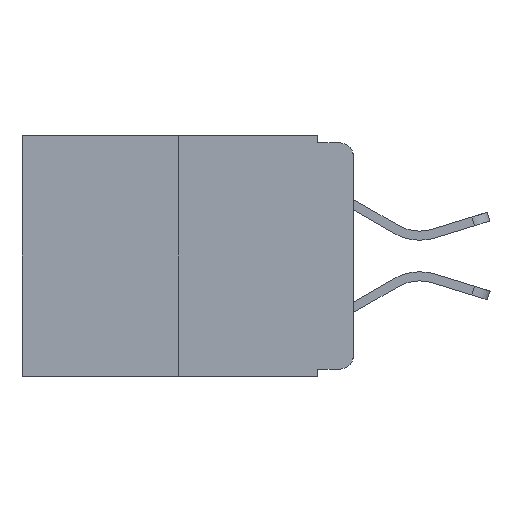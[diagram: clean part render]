
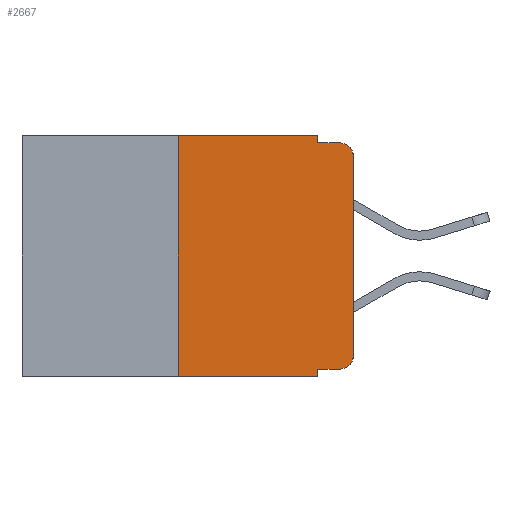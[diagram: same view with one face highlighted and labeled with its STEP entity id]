
A CAD part, left-side view. The second image highlights one B-rep face of the part: STEP entity #2667.
In plain terms, the highlighted planar face has unit normal (-1, 0, 0).
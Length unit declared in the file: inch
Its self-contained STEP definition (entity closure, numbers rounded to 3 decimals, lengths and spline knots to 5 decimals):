
#70 = ORIENTED_EDGE ( 'NONE', *, *, #11704, .T. ) ;
#273 = DIRECTION ( 'NONE',  ( -1., 0., 0. ) ) ;
#379 = CARTESIAN_POINT ( 'NONE',  ( 0., 0.02, -0.03 ) ) ;
#642 = CARTESIAN_POINT ( 'NONE',  ( 0., 0.051, -0.01 ) ) ;
#656 = LINE ( 'NONE', #13604, #9080 ) ;
#787 = CARTESIAN_POINT ( 'NONE',  ( 0., 0.25, -0.343 ) ) ;
#1092 = DIRECTION ( 'NONE',  ( 0., 0., -1. ) ) ;
#2587 = CARTESIAN_POINT ( 'NONE',  ( 0., 0.051, 0. ) ) ;
#2667 = ADVANCED_FACE ( 'NONE', ( #18910 ), #13984, .F. ) ;
#2803 = LINE ( 'NONE', #11101, #20347 ) ;
#3010 = LINE ( 'NONE', #6108, #13708 ) ;
#4211 = DIRECTION ( 'NONE',  ( 0., -1., 0. ) ) ;
#4557 = ORIENTED_EDGE ( 'NONE', *, *, #12743, .T. ) ;
#5712 = EDGE_CURVE ( 'NONE', #15341, #13823, #3010, .T. ) ;
#5773 = AXIS2_PLACEMENT_3D ( 'NONE', #379, #273, #9454 ) ;
#5851 = DIRECTION ( 'NONE',  ( 0., -1., 0. ) ) ;
#5857 = CARTESIAN_POINT ( 'NONE',  ( 0., 0., 0. ) ) ;
#6027 = DIRECTION ( 'NONE',  ( 1., 0., 0. ) ) ;
#6108 = CARTESIAN_POINT ( 'NONE',  ( 0., 0.051, 0. ) ) ;
#6131 = VECTOR ( 'NONE', #11629, 39.37008 ) ;
#6478 = CARTESIAN_POINT ( 'NONE',  ( 0., 0.051, 0. ) ) ;
#7147 = CIRCLE ( 'NONE', #5773, 0.02 ) ;
#7428 = CARTESIAN_POINT ( 'NONE',  ( 0., 0.051, -0.333 ) ) ;
#7812 = VERTEX_POINT ( 'NONE', #8791 ) ;
#8414 = VERTEX_POINT ( 'NONE', #18873 ) ;
#8791 = CARTESIAN_POINT ( 'NONE',  ( 0., 0.25, 0. ) ) ;
#8841 = EDGE_CURVE ( 'NONE', #7812, #15341, #656, .T. ) ;
#9080 = VECTOR ( 'NONE', #5851, 39.37008 ) ;
#9187 = DIRECTION ( 'NONE',  ( 0., 0., -1. ) ) ;
#9247 = LINE ( 'NONE', #5857, #9453 ) ;
#9311 = CARTESIAN_POINT ( 'NONE',  ( 0., 0.051, -0.343 ) ) ;
#9453 = VECTOR ( 'NONE', #15525, 39.37008 ) ;
#9454 = DIRECTION ( 'NONE',  ( 0., 0., -1. ) ) ;
#9625 = VERTEX_POINT ( 'NONE', #787 ) ;
#9995 = LINE ( 'NONE', #642, #15996 ) ;
#10186 = EDGE_CURVE ( 'NONE', #16521, #8414, #9247, .T. ) ;
#10545 = VERTEX_POINT ( 'NONE', #18075 ) ;
#11101 = CARTESIAN_POINT ( 'NONE',  ( 0., 0.473, -0.343 ) ) ;
#11535 = CIRCLE ( 'NONE', #18020, 0.02 ) ;
#11629 = DIRECTION ( 'NONE',  ( 0., 0., 1. ) ) ;
#11704 = EDGE_CURVE ( 'NONE', #9625, #18495, #2803, .T. ) ;
#11826 = CARTESIAN_POINT ( 'NONE',  ( 0., 0.02, -0.333 ) ) ;
#11968 = DIRECTION ( 'NONE',  ( 0., -1., 0. ) ) ;
#12009 = VERTEX_POINT ( 'NONE', #11826 ) ;
#12590 = CARTESIAN_POINT ( 'NONE',  ( 0., 0.473, 0. ) ) ;
#12743 = EDGE_CURVE ( 'NONE', #8414, #10545, #7147, .T. ) ;
#12933 = ORIENTED_EDGE ( 'NONE', *, *, #17542, .F. ) ;
#12995 = CARTESIAN_POINT ( 'NONE',  ( 0., 0.25, 0. ) ) ;
#13089 = EDGE_LOOP ( 'NONE', ( #16188, #4557, #18526, #14894, #14012, #13442, #70, #12933, #13584, #18326 ) ) ;
#13279 = DIRECTION ( 'NONE',  ( 0., 0., -1. ) ) ;
#13442 = ORIENTED_EDGE ( 'NONE', *, *, #17263, .F. ) ;
#13584 = ORIENTED_EDGE ( 'NONE', *, *, #15685, .T. ) ;
#13587 = EDGE_CURVE ( 'NONE', #12009, #16521, #11535, .T. ) ;
#13604 = CARTESIAN_POINT ( 'NONE',  ( 0., 0.473, 0. ) ) ;
#13708 = VECTOR ( 'NONE', #9187, 39.37008 ) ;
#13823 = VERTEX_POINT ( 'NONE', #17540 ) ;
#13984 = PLANE ( 'NONE',  #19229 ) ;
#14012 = ORIENTED_EDGE ( 'NONE', *, *, #8841, .F. ) ;
#14894 = ORIENTED_EDGE ( 'NONE', *, *, #5712, .F. ) ;
#15341 = VERTEX_POINT ( 'NONE', #6478 ) ;
#15378 = CARTESIAN_POINT ( 'NONE',  ( 0., 0.051, -0.333 ) ) ;
#15525 = DIRECTION ( 'NONE',  ( 0., 0., 1. ) ) ;
#15685 = EDGE_CURVE ( 'NONE', #20775, #12009, #18591, .T. ) ;
#15996 = VECTOR ( 'NONE', #19799, 39.37008 ) ;
#16183 = DIRECTION ( 'NONE',  ( -1., 0., 0. ) ) ;
#16188 = ORIENTED_EDGE ( 'NONE', *, *, #10186, .T. ) ;
#16521 = VERTEX_POINT ( 'NONE', #20102 ) ;
#17181 = LINE ( 'NONE', #2587, #17692 ) ;
#17263 = EDGE_CURVE ( 'NONE', #9625, #7812, #19626, .T. ) ;
#17540 = CARTESIAN_POINT ( 'NONE',  ( 0., 0.051, -0.01 ) ) ;
#17542 = EDGE_CURVE ( 'NONE', #20775, #18495, #17181, .T. ) ;
#17692 = VECTOR ( 'NONE', #1092, 39.37008 ) ;
#17972 = VECTOR ( 'NONE', #11968, 39.37008 ) ;
#17996 = CARTESIAN_POINT ( 'NONE',  ( 0., 0.02, -0.313 ) ) ;
#18020 = AXIS2_PLACEMENT_3D ( 'NONE', #17996, #16183, #13279 ) ;
#18075 = CARTESIAN_POINT ( 'NONE',  ( 0., 0.02, -0.01 ) ) ;
#18326 = ORIENTED_EDGE ( 'NONE', *, *, #13587, .T. ) ;
#18495 = VERTEX_POINT ( 'NONE', #9311 ) ;
#18526 = ORIENTED_EDGE ( 'NONE', *, *, #19641, .F. ) ;
#18591 = LINE ( 'NONE', #15378, #17972 ) ;
#18873 = CARTESIAN_POINT ( 'NONE',  ( 0., 0., -0.03 ) ) ;
#18910 = FACE_OUTER_BOUND ( 'NONE', #13089, .T. ) ;
#19115 = DIRECTION ( 'NONE',  ( 0., 0., -1. ) ) ;
#19229 = AXIS2_PLACEMENT_3D ( 'NONE', #12590, #6027, #19115 ) ;
#19626 = LINE ( 'NONE', #12995, #6131 ) ;
#19641 = EDGE_CURVE ( 'NONE', #13823, #10545, #9995, .T. ) ;
#19799 = DIRECTION ( 'NONE',  ( 0., -1., 0. ) ) ;
#20102 = CARTESIAN_POINT ( 'NONE',  ( 0., 0., -0.313 ) ) ;
#20347 = VECTOR ( 'NONE', #4211, 39.37008 ) ;
#20775 = VERTEX_POINT ( 'NONE', #7428 ) ;
